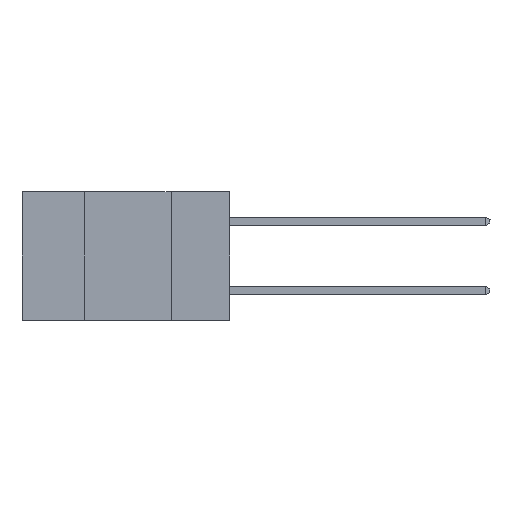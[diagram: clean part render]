
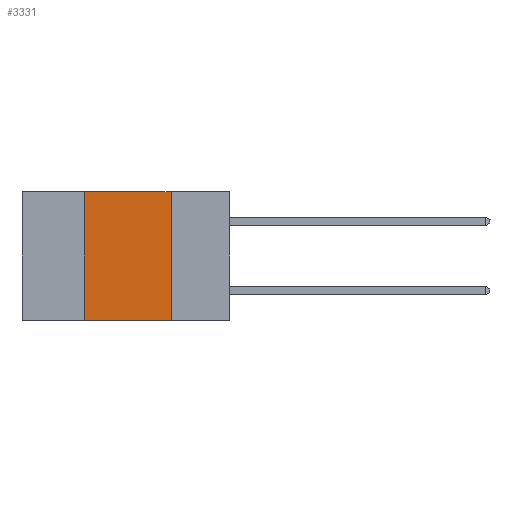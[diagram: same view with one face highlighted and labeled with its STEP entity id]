
A CAD part, left-side view. The second image highlights one B-rep face of the part: STEP entity #3331.
In plain terms, the highlighted planar face has unit normal (-1, 0, 0).
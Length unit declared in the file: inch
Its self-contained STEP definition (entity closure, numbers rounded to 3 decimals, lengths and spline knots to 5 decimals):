
#419 = CARTESIAN_POINT ( 'NONE',  ( 0., 0.42, -0.37 ) ) ;
#524 = ORIENTED_EDGE ( 'NONE', *, *, #4606, .F. ) ;
#905 = CARTESIAN_POINT ( 'NONE',  ( 0., 0.42, 0. ) ) ;
#1484 = EDGE_CURVE ( 'NONE', #4594, #5417, #5588, .T. ) ;
#2039 = DIRECTION ( 'NONE',  ( 0., 0., -1. ) ) ;
#2214 = DIRECTION ( 'NONE',  ( 0., -1., 0. ) ) ;
#2673 = CARTESIAN_POINT ( 'NONE',  ( 0., 0.6, 0. ) ) ;
#3331 = ADVANCED_FACE ( 'NONE', ( #7094 ), #10586, .F. ) ;
#3669 = VERTEX_POINT ( 'NONE', #9671 ) ;
#3857 = EDGE_CURVE ( 'NONE', #5417, #3669, #8119, .T. ) ;
#3911 = ORIENTED_EDGE ( 'NONE', *, *, #3857, .F. ) ;
#4254 = VECTOR ( 'NONE', #9901, 39.37008 ) ;
#4298 = EDGE_CURVE ( 'NONE', #4594, #7413, #7440, .T. ) ;
#4594 = VERTEX_POINT ( 'NONE', #9900 ) ;
#4606 = EDGE_CURVE ( 'NONE', #3669, #7413, #6315, .T. ) ;
#4697 = CARTESIAN_POINT ( 'NONE',  ( 0., 0.6, 0. ) ) ;
#4954 = VECTOR ( 'NONE', #2039, 39.37008 ) ;
#4985 = VECTOR ( 'NONE', #8142, 39.37008 ) ;
#5356 = DIRECTION ( 'NONE',  ( 1., 0., 0. ) ) ;
#5417 = VERTEX_POINT ( 'NONE', #905 ) ;
#5559 = ORIENTED_EDGE ( 'NONE', *, *, #1484, .F. ) ;
#5588 = LINE ( 'NONE', #419, #4985 ) ;
#5691 = ORIENTED_EDGE ( 'NONE', *, *, #4298, .T. ) ;
#6219 = VECTOR ( 'NONE', #2214, 39.37008 ) ;
#6315 = LINE ( 'NONE', #8173, #4954 ) ;
#7094 = FACE_OUTER_BOUND ( 'NONE', #10813, .T. ) ;
#7413 = VERTEX_POINT ( 'NONE', #7677 ) ;
#7440 = LINE ( 'NONE', #10134, #6219 ) ;
#7677 = CARTESIAN_POINT ( 'NONE',  ( 0., 0.17, -0.37 ) ) ;
#8119 = LINE ( 'NONE', #4697, #4254 ) ;
#8142 = DIRECTION ( 'NONE',  ( 0., 0., 1. ) ) ;
#8173 = CARTESIAN_POINT ( 'NONE',  ( 0., 0.17, -0.37 ) ) ;
#8184 = DIRECTION ( 'NONE',  ( 0., 0., -1. ) ) ;
#8557 = AXIS2_PLACEMENT_3D ( 'NONE', #2673, #5356, #8184 ) ;
#9671 = CARTESIAN_POINT ( 'NONE',  ( 0., 0.17, 0. ) ) ;
#9900 = CARTESIAN_POINT ( 'NONE',  ( 0., 0.42, -0.37 ) ) ;
#9901 = DIRECTION ( 'NONE',  ( 0., -1., 0. ) ) ;
#10134 = CARTESIAN_POINT ( 'NONE',  ( 0., 0.6, -0.37 ) ) ;
#10586 = PLANE ( 'NONE',  #8557 ) ;
#10813 = EDGE_LOOP ( 'NONE', ( #524, #3911, #5559, #5691 ) ) ;
